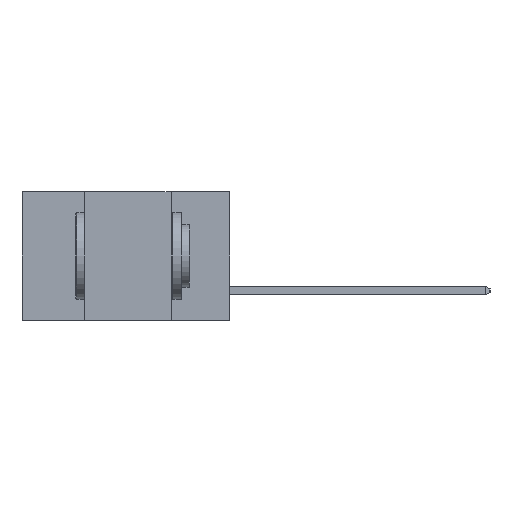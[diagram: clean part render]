
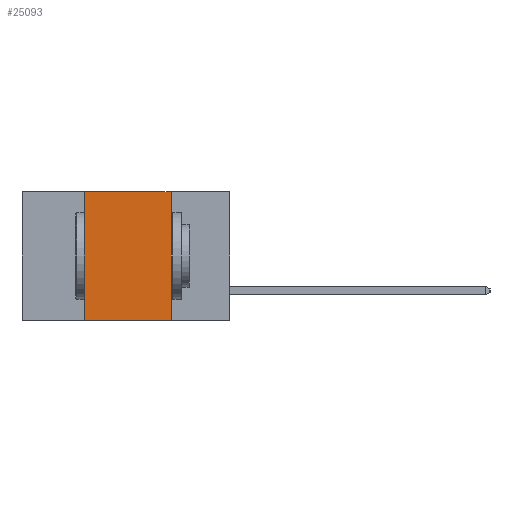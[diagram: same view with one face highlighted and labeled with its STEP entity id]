
A CAD part, left-side view. The second image highlights one B-rep face of the part: STEP entity #25093.
In plain terms, the highlighted planar face has unit normal (-1, 0, 0).
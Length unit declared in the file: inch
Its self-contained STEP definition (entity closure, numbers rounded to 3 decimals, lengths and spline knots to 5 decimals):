
#214 = LINE ( 'NONE', #8822, #12691 ) ;
#1334 = ORIENTED_EDGE ( 'NONE', *, *, #8030, .F. ) ;
#5164 = VERTEX_POINT ( 'NONE', #22186 ) ;
#6535 = ORIENTED_EDGE ( 'NONE', *, *, #18796, .T. ) ;
#7215 = DIRECTION ( 'NONE',  ( 0., 0., -1. ) ) ;
#7220 = VECTOR ( 'NONE', #7215, 39.37008 ) ;
#7438 = DIRECTION ( 'NONE',  ( 0., 0., 1. ) ) ;
#7857 = CARTESIAN_POINT ( 'NONE',  ( 0., 0.6, -0.37 ) ) ;
#8030 = EDGE_CURVE ( 'NONE', #26886, #9894, #214, .T. ) ;
#8822 = CARTESIAN_POINT ( 'NONE',  ( 0., 0.6, 0. ) ) ;
#8989 = DIRECTION ( 'NONE',  ( 1., 0., 0. ) ) ;
#9589 = CARTESIAN_POINT ( 'NONE',  ( 0., 0.17, 0. ) ) ;
#9894 = VERTEX_POINT ( 'NONE', #28730 ) ;
#11528 = ORIENTED_EDGE ( 'NONE', *, *, #16623, .F. ) ;
#12126 = VERTEX_POINT ( 'NONE', #31404 ) ;
#12691 = VECTOR ( 'NONE', #23581, 39.37008 ) ;
#13205 = EDGE_LOOP ( 'NONE', ( #26432, #1334, #11528, #6535 ) ) ;
#14011 = VECTOR ( 'NONE', #27540, 39.37008 ) ;
#14795 = LINE ( 'NONE', #7857, #14011 ) ;
#15287 = AXIS2_PLACEMENT_3D ( 'NONE', #30932, #8989, #26195 ) ;
#16550 = EDGE_CURVE ( 'NONE', #9894, #12126, #26869, .T. ) ;
#16623 = EDGE_CURVE ( 'NONE', #5164, #26886, #25301, .T. ) ;
#18796 = EDGE_CURVE ( 'NONE', #5164, #12126, #14795, .T. ) ;
#19746 = CARTESIAN_POINT ( 'NONE',  ( 0., 0.42, 0. ) ) ;
#22186 = CARTESIAN_POINT ( 'NONE',  ( 0., 0.42, -0.37 ) ) ;
#22504 = FACE_OUTER_BOUND ( 'NONE', #13205, .T. ) ;
#23581 = DIRECTION ( 'NONE',  ( 0., -1., 0. ) ) ;
#23742 = PLANE ( 'NONE',  #15287 ) ;
#24569 = VECTOR ( 'NONE', #7438, 39.37008 ) ;
#25093 = ADVANCED_FACE ( 'NONE', ( #22504 ), #23742, .F. ) ;
#25301 = LINE ( 'NONE', #19746, #24569 ) ;
#26195 = DIRECTION ( 'NONE',  ( 0., 0., -1. ) ) ;
#26432 = ORIENTED_EDGE ( 'NONE', *, *, #16550, .F. ) ;
#26869 = LINE ( 'NONE', #9589, #7220 ) ;
#26886 = VERTEX_POINT ( 'NONE', #30513 ) ;
#27540 = DIRECTION ( 'NONE',  ( 0., -1., 0. ) ) ;
#28730 = CARTESIAN_POINT ( 'NONE',  ( 0., 0.17, 0. ) ) ;
#30513 = CARTESIAN_POINT ( 'NONE',  ( 0., 0.42, 0. ) ) ;
#30932 = CARTESIAN_POINT ( 'NONE',  ( 0., 0.6, 0. ) ) ;
#31404 = CARTESIAN_POINT ( 'NONE',  ( 0., 0.17, -0.37 ) ) ;
